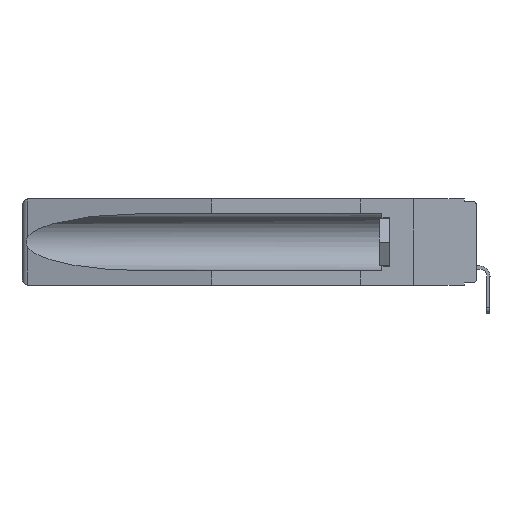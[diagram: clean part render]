
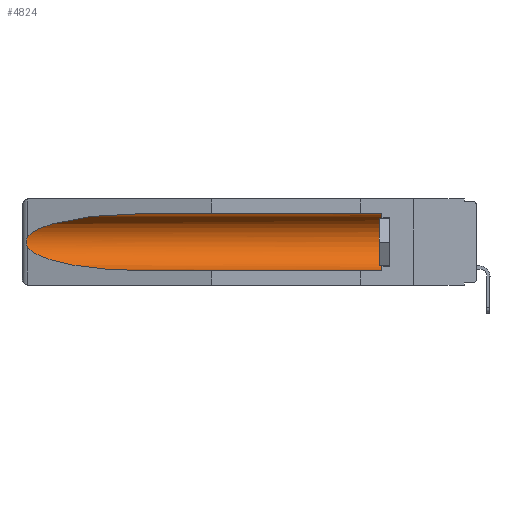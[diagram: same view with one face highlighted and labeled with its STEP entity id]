
A CAD part, left-side view. The second image highlights one B-rep face of the part: STEP entity #4824.
In plain terms, the highlighted cylindrical face has radius 2.857 mm (diameter 5.715 mm), a partial arc.
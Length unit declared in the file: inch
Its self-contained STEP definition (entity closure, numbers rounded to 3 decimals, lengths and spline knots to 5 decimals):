
#6 = EDGE_CURVE ( 'NONE', #9394, #12380, #9662, .T. ) ;
#224 = VERTEX_POINT ( 'NONE', #5350 ) ;
#631 = CARTESIAN_POINT ( 'NONE',  ( 0.155, 1.07973, -0.059 ) ) ;
#701 = CARTESIAN_POINT ( 'NONE',  ( 0.155, 1.07973, -0.284 ) ) ;
#942 = CARTESIAN_POINT ( 'NONE',  ( 0.2673, 1.5327, -0.16383 ) ) ;
#1030 = CARTESIAN_POINT ( 'NONE',  ( 0.155, -0.30754, -0.059 ) ) ;
#1510 = AXIS2_PLACEMENT_3D ( 'NONE', #4258, #10278, #14996 ) ;
#2028 = CARTESIAN_POINT ( 'NONE',  ( 0.26537, 1.52718, -0.19328 ) ) ;
#2474 = CARTESIAN_POINT ( 'NONE',  ( 0.155, 0.126, -0.1715 ) ) ;
#2536 = LINE ( 'NONE', #19221, #3051 ) ;
#2622 = CARTESIAN_POINT ( 'NONE',  ( 0.26537, 1.52718, -0.14972 ) ) ;
#2801 = VERTEX_POINT ( 'NONE', #8775 ) ;
#3051 = VECTOR ( 'NONE', #3830, 39.37008 ) ;
#3287 = EDGE_CURVE ( 'NONE', #11076, #9623, #8801, .T. ) ;
#3695 = EDGE_CURVE ( 'NONE', #2801, #11076, #13438, .T. ) ;
#3830 = DIRECTION ( 'NONE',  ( 0., 1., 0. ) ) ;
#4258 = CARTESIAN_POINT ( 'NONE',  ( 0.155, -0.30754, -0.1715 ) ) ;
#4824 = ADVANCED_FACE ( 'NONE', ( #14713 ), #17780, .F. ) ;
#4854 = CARTESIAN_POINT ( 'NONE',  ( 0.26537, 1.52718, -0.14972 ) ) ;
#5350 = CARTESIAN_POINT ( 'NONE',  ( 0.155, 0.126, -0.284 ) ) ;
#5552 = EDGE_CURVE ( 'NONE', #224, #12380, #2536, .T. ) ;
#6733 = EDGE_LOOP ( 'NONE', ( #7655, #14460, #17620, #8061, #8388, #18703 ) ) ;
#6980 = CARTESIAN_POINT ( 'NONE',  ( 0.26655, 1.53094, -0.18657 ) ) ;
#7414 = CARTESIAN_POINT ( 'NONE',  ( 0.26537, 1.52718, -0.19328 ) ) ;
#7546 = CARTESIAN_POINT ( 'NONE',  ( 0.21114, 1.30732, -0.059 ) ) ;
#7655 = ORIENTED_EDGE ( 'NONE', *, *, #3287, .T. ) ;
#8061 = ORIENTED_EDGE ( 'NONE', *, *, #5552, .F. ) ;
#8388 = ORIENTED_EDGE ( 'NONE', *, *, #8518, .T. ) ;
#8518 = EDGE_CURVE ( 'NONE', #224, #2801, #14527, .T. ) ;
#8645 = CARTESIAN_POINT ( 'NONE',  ( 0.26597, 1.52961, -0.15275 ) ) ;
#8741 = CARTESIAN_POINT ( 'NONE',  ( 0.2673, 1.53269, -0.17917 ) ) ;
#8775 = CARTESIAN_POINT ( 'NONE',  ( 0.155, 0.126, -0.059 ) ) ;
#8801 =( BOUNDED_CURVE ( )  B_SPLINE_CURVE ( 3, ( #9327, #7546, #15233, #15133 ),
 .UNSPECIFIED., .F., .T. ) 
 B_SPLINE_CURVE_WITH_KNOTS ( ( 4, 4 ),
 ( 4.71239, 6.08839 ),
 .UNSPECIFIED. ) 
 CURVE ( )  GEOMETRIC_REPRESENTATION_ITEM ( )  RATIONAL_B_SPLINE_CURVE ( ( 1., 0.848, 0.848, 1. ) ) 
 REPRESENTATION_ITEM ( '' )  );
#8835 = CARTESIAN_POINT ( 'NONE',  ( 0.26597, 1.5296, -0.19026 ) ) ;
#9327 = CARTESIAN_POINT ( 'NONE',  ( 0.155, 1.07973, -0.059 ) ) ;
#9394 = VERTEX_POINT ( 'NONE', #7414 ) ;
#9623 = VERTEX_POINT ( 'NONE', #4854 ) ;
#9662 =( BOUNDED_CURVE ( )  B_SPLINE_CURVE ( 3, ( #2028, #17310, #16916, #14154 ),
 .UNSPECIFIED., .F., .F. ) 
 B_SPLINE_CURVE_WITH_KNOTS ( ( 4, 4 ),
 ( 0.1948, 1.5708 ),
 .UNSPECIFIED. ) 
 CURVE ( )  GEOMETRIC_REPRESENTATION_ITEM ( )  RATIONAL_B_SPLINE_CURVE ( ( 1., 0.848, 0.848, 1. ) ) 
 REPRESENTATION_ITEM ( '' )  );
#10216 = CARTESIAN_POINT ( 'NONE',  ( 0.26537, 1.52718, -0.19328 ) ) ;
#10278 = DIRECTION ( 'NONE',  ( 0., 1., 0. ) ) ;
#11076 = VERTEX_POINT ( 'NONE', #631 ) ;
#12380 = VERTEX_POINT ( 'NONE', #701 ) ;
#13430 = B_SPLINE_CURVE_WITH_KNOTS ( 'NONE', 3,
 ( #2622, #8645, #14651, #942, #14555, #17715, #8741, #6980, #8835, #10216 ),
 .UNSPECIFIED., .F., .F.,
 ( 4, 2, 2, 2, 4 ),
 ( 0., 0.00029, 0.00058, 0.00087, 0.00117 ),
 .UNSPECIFIED. ) ;
#13438 = LINE ( 'NONE', #1030, #17860 ) ;
#13575 = AXIS2_PLACEMENT_3D ( 'NONE', #2474, #16083, #17366 ) ;
#14154 = CARTESIAN_POINT ( 'NONE',  ( 0.155, 1.07973, -0.284 ) ) ;
#14460 = ORIENTED_EDGE ( 'NONE', *, *, #15770, .T. ) ;
#14527 = CIRCLE ( 'NONE', #13575, 0.1125 ) ;
#14539 = DIRECTION ( 'NONE',  ( 0., 1., 0. ) ) ;
#14555 = CARTESIAN_POINT ( 'NONE',  ( 0.2675, 1.53308, -0.16763 ) ) ;
#14651 = CARTESIAN_POINT ( 'NONE',  ( 0.26654, 1.53092, -0.15636 ) ) ;
#14713 = FACE_OUTER_BOUND ( 'NONE', #6733, .T. ) ;
#14996 = DIRECTION ( 'NONE',  ( 0., 0., 1. ) ) ;
#15133 = CARTESIAN_POINT ( 'NONE',  ( 0.26537, 1.52718, -0.14972 ) ) ;
#15233 = CARTESIAN_POINT ( 'NONE',  ( 0.25451, 1.48313, -0.09465 ) ) ;
#15770 = EDGE_CURVE ( 'NONE', #9623, #9394, #13430, .T. ) ;
#16083 = DIRECTION ( 'NONE',  ( 0., -1., 0. ) ) ;
#16916 = CARTESIAN_POINT ( 'NONE',  ( 0.21114, 1.30732, -0.284 ) ) ;
#17310 = CARTESIAN_POINT ( 'NONE',  ( 0.25451, 1.48313, -0.24835 ) ) ;
#17366 = DIRECTION ( 'NONE',  ( 0., 0., 1. ) ) ;
#17620 = ORIENTED_EDGE ( 'NONE', *, *, #6, .T. ) ;
#17715 = CARTESIAN_POINT ( 'NONE',  ( 0.2675, 1.53308, -0.17534 ) ) ;
#17780 = CYLINDRICAL_SURFACE ( 'NONE', #1510, 0.1125 ) ;
#17860 = VECTOR ( 'NONE', #14539, 39.37008 ) ;
#18703 = ORIENTED_EDGE ( 'NONE', *, *, #3695, .T. ) ;
#19221 = CARTESIAN_POINT ( 'NONE',  ( 0.155, -0.30754, -0.284 ) ) ;
